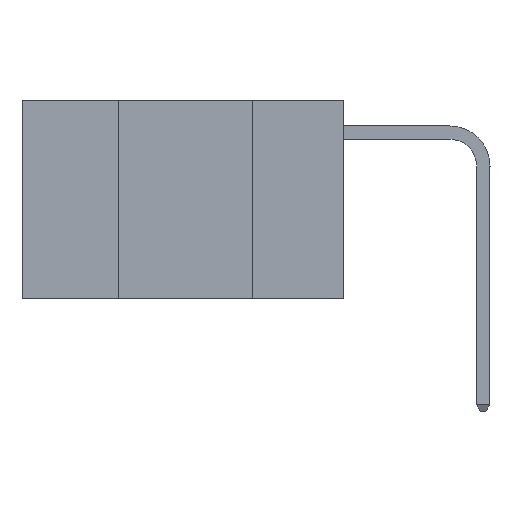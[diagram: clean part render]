
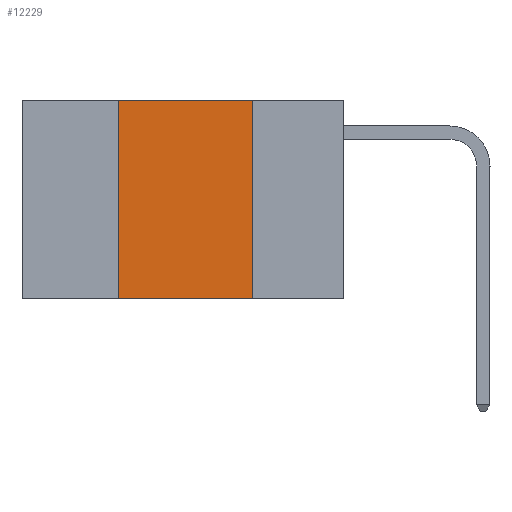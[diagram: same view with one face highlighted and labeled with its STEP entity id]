
A CAD part, left-side view. The second image highlights one B-rep face of the part: STEP entity #12229.
In plain terms, the highlighted planar face has unit normal (-1, 0, 0).
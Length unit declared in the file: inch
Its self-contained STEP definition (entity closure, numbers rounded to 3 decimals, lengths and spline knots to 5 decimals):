
#1 = VERTEX_POINT ( 'NONE', #577 ) ;
#83 = CARTESIAN_POINT ( 'NONE',  ( 0., 0.17, 0. ) ) ;
#115 = ORIENTED_EDGE ( 'NONE', *, *, #11918, .T. ) ;
#231 = LINE ( 'NONE', #4022, #5646 ) ;
#577 = CARTESIAN_POINT ( 'NONE',  ( 0., 0.42, -0.37 ) ) ;
#780 = DIRECTION ( 'NONE',  ( 0., -1., 0. ) ) ;
#873 = VERTEX_POINT ( 'NONE', #4192 ) ;
#1602 = CARTESIAN_POINT ( 'NONE',  ( 0., 0.6, 0. ) ) ;
#2526 = ORIENTED_EDGE ( 'NONE', *, *, #2998, .F. ) ;
#2538 = VERTEX_POINT ( 'NONE', #7089 ) ;
#2998 = EDGE_CURVE ( 'NONE', #873, #2538, #7749, .T. ) ;
#3654 = DIRECTION ( 'NONE',  ( 1., 0., 0. ) ) ;
#4022 = CARTESIAN_POINT ( 'NONE',  ( 0., 0.42, 0. ) ) ;
#4192 = CARTESIAN_POINT ( 'NONE',  ( 0., 0.42, 0. ) ) ;
#5043 = LINE ( 'NONE', #83, #8301 ) ;
#5646 = VECTOR ( 'NONE', #10939, 39.37008 ) ;
#7089 = CARTESIAN_POINT ( 'NONE',  ( 0., 0.17, 0. ) ) ;
#7147 = CARTESIAN_POINT ( 'NONE',  ( 0., 0.6, -0.37 ) ) ;
#7638 = PLANE ( 'NONE',  #12680 ) ;
#7666 = VECTOR ( 'NONE', #8131, 39.37008 ) ;
#7749 = LINE ( 'NONE', #7842, #12300 ) ;
#7842 = CARTESIAN_POINT ( 'NONE',  ( 0., 0.6, 0. ) ) ;
#8131 = DIRECTION ( 'NONE',  ( 0., -1., 0. ) ) ;
#8301 = VECTOR ( 'NONE', #9116, 39.37008 ) ;
#8599 = VERTEX_POINT ( 'NONE', #11711 ) ;
#8819 = EDGE_LOOP ( 'NONE', ( #10171, #2526, #10463, #115 ) ) ;
#9116 = DIRECTION ( 'NONE',  ( 0., 0., -1. ) ) ;
#10171 = ORIENTED_EDGE ( 'NONE', *, *, #10872, .F. ) ;
#10260 = LINE ( 'NONE', #7147, #7666 ) ;
#10463 = ORIENTED_EDGE ( 'NONE', *, *, #11347, .F. ) ;
#10581 = DIRECTION ( 'NONE',  ( 0., 0., -1. ) ) ;
#10872 = EDGE_CURVE ( 'NONE', #2538, #8599, #5043, .T. ) ;
#10939 = DIRECTION ( 'NONE',  ( 0., 0., 1. ) ) ;
#11347 = EDGE_CURVE ( 'NONE', #1, #873, #231, .T. ) ;
#11711 = CARTESIAN_POINT ( 'NONE',  ( 0., 0.17, -0.37 ) ) ;
#11768 = FACE_OUTER_BOUND ( 'NONE', #8819, .T. ) ;
#11918 = EDGE_CURVE ( 'NONE', #1, #8599, #10260, .T. ) ;
#12229 = ADVANCED_FACE ( 'NONE', ( #11768 ), #7638, .F. ) ;
#12300 = VECTOR ( 'NONE', #780, 39.37008 ) ;
#12680 = AXIS2_PLACEMENT_3D ( 'NONE', #1602, #3654, #10581 ) ;
